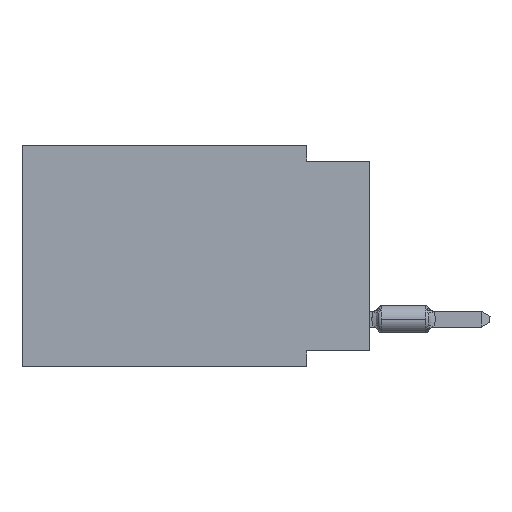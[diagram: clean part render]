
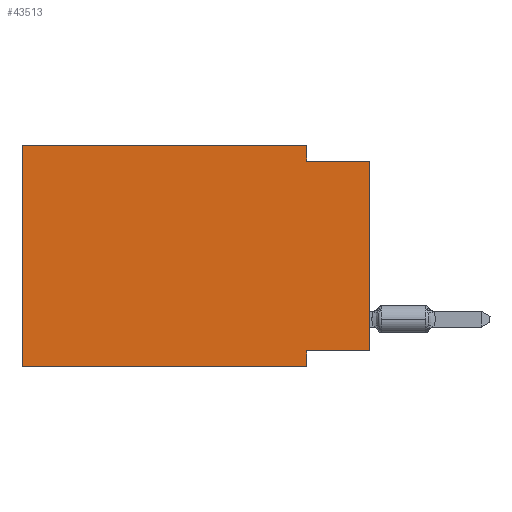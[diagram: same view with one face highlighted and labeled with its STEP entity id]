
A CAD part, left-side view. The second image highlights one B-rep face of the part: STEP entity #43513.
In plain terms, the highlighted planar face has unit normal (-1, 0, 0).
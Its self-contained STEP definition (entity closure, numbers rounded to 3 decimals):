
#2304 = CARTESIAN_POINT ( 'NONE',  ( 0., 13.97, 0. ) ) ;
#4319 = LINE ( 'NONE', #14718, #77364 ) ;
#8216 = LINE ( 'NONE', #51744, #12841 ) ;
#9203 = VERTEX_POINT ( 'NONE', #18630 ) ;
#9761 = LINE ( 'NONE', #69544, #101272 ) ;
#11420 = EDGE_CURVE ( 'NONE', #99433, #39467, #8216, .T. ) ;
#12841 = VECTOR ( 'NONE', #24466, 1000. ) ;
#14703 = VERTEX_POINT ( 'NONE', #101419 ) ;
#14718 = CARTESIAN_POINT ( 'NONE',  ( 0., 0., -8.255 ) ) ;
#16710 = AXIS2_PLACEMENT_3D ( 'NONE', #110749, #19840, #45399 ) ;
#17941 = VECTOR ( 'NONE', #63256, 1000. ) ;
#18630 = CARTESIAN_POINT ( 'NONE',  ( 0., 13.97, -8.89 ) ) ;
#19102 = ORIENTED_EDGE ( 'NONE', *, *, #11420, .F. ) ;
#19840 = DIRECTION ( 'NONE',  ( 1., 0., 0. ) ) ;
#19934 = VERTEX_POINT ( 'NONE', #94652 ) ;
#21043 = EDGE_CURVE ( 'NONE', #39467, #34395, #102630, .T. ) ;
#22314 = ORIENTED_EDGE ( 'NONE', *, *, #21043, .F. ) ;
#24466 = DIRECTION ( 'NONE',  ( 0., 0., -1. ) ) ;
#26679 = CARTESIAN_POINT ( 'NONE',  ( 0., 0., 0. ) ) ;
#29716 = DIRECTION ( 'NONE',  ( 0., -1., 0. ) ) ;
#30576 = EDGE_CURVE ( 'NONE', #9203, #14703, #9761, .T. ) ;
#32882 = VERTEX_POINT ( 'NONE', #100096 ) ;
#34233 = DIRECTION ( 'NONE',  ( 0., 0., 1. ) ) ;
#34325 = EDGE_CURVE ( 'NONE', #9203, #64045, #38988, .T. ) ;
#34395 = VERTEX_POINT ( 'NONE', #73837 ) ;
#38988 = LINE ( 'NONE', #83684, #106022 ) ;
#39377 = PLANE ( 'NONE',  #16710 ) ;
#39467 = VERTEX_POINT ( 'NONE', #101475 ) ;
#41394 = DIRECTION ( 'NONE',  ( 0., 1., 0. ) ) ;
#43513 = ADVANCED_FACE ( 'NONE', ( #99347 ), #39377, .F. ) ;
#44575 = CARTESIAN_POINT ( 'NONE',  ( 0., 2.54, -8.89 ) ) ;
#45399 = DIRECTION ( 'NONE',  ( 0., 0., -1. ) ) ;
#47330 = EDGE_CURVE ( 'NONE', #14703, #99433, #55675, .T. ) ;
#48173 = ORIENTED_EDGE ( 'NONE', *, *, #76583, .F. ) ;
#51744 = CARTESIAN_POINT ( 'NONE',  ( 0., 2.54, 0. ) ) ;
#51915 = CARTESIAN_POINT ( 'NONE',  ( 0., 2.54, -8.89 ) ) ;
#52824 = LINE ( 'NONE', #26679, #86152 ) ;
#53476 = ORIENTED_EDGE ( 'NONE', *, *, #68970, .F. ) ;
#55675 = LINE ( 'NONE', #2304, #17941 ) ;
#57468 = CARTESIAN_POINT ( 'NONE',  ( 0., 2.54, 0. ) ) ;
#57981 = CARTESIAN_POINT ( 'NONE',  ( 0., 0., -0.635 ) ) ;
#60839 = VECTOR ( 'NONE', #102063, 1000. ) ;
#63256 = DIRECTION ( 'NONE',  ( 0., -1., 0. ) ) ;
#64045 = VERTEX_POINT ( 'NONE', #44575 ) ;
#66251 = EDGE_CURVE ( 'NONE', #19934, #34395, #52824, .T. ) ;
#68970 = EDGE_CURVE ( 'NONE', #32882, #64045, #112840, .T. ) ;
#69544 = CARTESIAN_POINT ( 'NONE',  ( 0., 13.97, 0. ) ) ;
#70392 = EDGE_LOOP ( 'NONE', ( #91888, #22314, #19102, #95080, #113700, #77287, #53476, #48173 ) ) ;
#73837 = CARTESIAN_POINT ( 'NONE',  ( 0., 0., -0.635 ) ) ;
#76583 = EDGE_CURVE ( 'NONE', #19934, #32882, #4319, .T. ) ;
#77287 = ORIENTED_EDGE ( 'NONE', *, *, #34325, .T. ) ;
#77364 = VECTOR ( 'NONE', #41394, 1000. ) ;
#83684 = CARTESIAN_POINT ( 'NONE',  ( 0., 13.97, -8.89 ) ) ;
#86145 = DIRECTION ( 'NONE',  ( 0., 0., -1. ) ) ;
#86152 = VECTOR ( 'NONE', #34233, 1000. ) ;
#91888 = ORIENTED_EDGE ( 'NONE', *, *, #66251, .T. ) ;
#92104 = VECTOR ( 'NONE', #86145, 1000. ) ;
#94652 = CARTESIAN_POINT ( 'NONE',  ( 0., 0., -8.255 ) ) ;
#95080 = ORIENTED_EDGE ( 'NONE', *, *, #47330, .F. ) ;
#99347 = FACE_OUTER_BOUND ( 'NONE', #70392, .T. ) ;
#99433 = VERTEX_POINT ( 'NONE', #57468 ) ;
#100096 = CARTESIAN_POINT ( 'NONE',  ( 0., 2.54, -8.255 ) ) ;
#101272 = VECTOR ( 'NONE', #106647, 1000. ) ;
#101419 = CARTESIAN_POINT ( 'NONE',  ( 0., 13.97, 0. ) ) ;
#101475 = CARTESIAN_POINT ( 'NONE',  ( 0., 2.54, -0.635 ) ) ;
#102063 = DIRECTION ( 'NONE',  ( 0., -1., 0. ) ) ;
#102630 = LINE ( 'NONE', #57981, #60839 ) ;
#106022 = VECTOR ( 'NONE', #29716, 1000. ) ;
#106647 = DIRECTION ( 'NONE',  ( 0., 0., 1. ) ) ;
#110749 = CARTESIAN_POINT ( 'NONE',  ( 0., 13.97, 0. ) ) ;
#112840 = LINE ( 'NONE', #51915, #92104 ) ;
#113700 = ORIENTED_EDGE ( 'NONE', *, *, #30576, .F. ) ;
